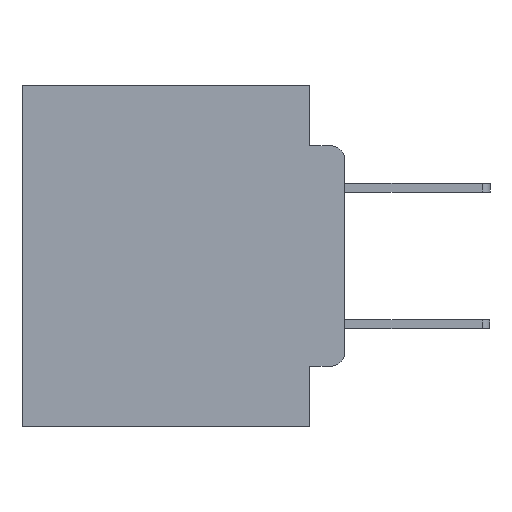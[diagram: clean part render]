
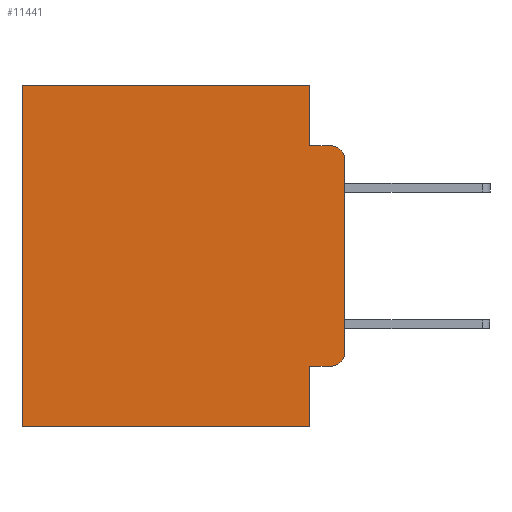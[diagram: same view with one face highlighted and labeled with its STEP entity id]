
A CAD part, left-side view. The second image highlights one B-rep face of the part: STEP entity #11441.
In plain terms, the highlighted planar face has unit normal (-1, 0, 0).
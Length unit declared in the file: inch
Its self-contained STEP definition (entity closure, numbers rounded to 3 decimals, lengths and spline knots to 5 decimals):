
#386 = VECTOR ( 'NONE', #3322, 39.37008 ) ;
#460 = AXIS2_PLACEMENT_3D ( 'NONE', #9773, #25426, #12042 ) ;
#721 = DIRECTION ( 'NONE',  ( 1., 0., 0. ) ) ;
#791 = ORIENTED_EDGE ( 'NONE', *, *, #3352, .T. ) ;
#1044 = DIRECTION ( 'NONE',  ( 0., 0., -1. ) ) ;
#1881 = DIRECTION ( 'NONE',  ( 0., -1., 0. ) ) ;
#1906 = DIRECTION ( 'NONE',  ( 0., 1., 0. ) ) ;
#2902 = ORIENTED_EDGE ( 'NONE', *, *, #4835, .T. ) ;
#3322 = DIRECTION ( 'NONE',  ( 0., -1., 0. ) ) ;
#3352 = EDGE_CURVE ( 'NONE', #27352, #16825, #17367, .T. ) ;
#3457 = VECTOR ( 'NONE', #28749, 39.37008 ) ;
#3898 = DIRECTION ( 'NONE',  ( 0., 0., -1. ) ) ;
#4165 = LINE ( 'NONE', #27867, #21397 ) ;
#4477 = VERTEX_POINT ( 'NONE', #10609 ) ;
#4835 = EDGE_CURVE ( 'NONE', #21523, #27352, #12340, .T. ) ;
#5110 = CARTESIAN_POINT ( 'NONE',  ( 0.298, 0., 0. ) ) ;
#5641 = ORIENTED_EDGE ( 'NONE', *, *, #12395, .F. ) ;
#6027 = ORIENTED_EDGE ( 'NONE', *, *, #15398, .T. ) ;
#6313 = VERTEX_POINT ( 'NONE', #15136 ) ;
#6376 = EDGE_CURVE ( 'NONE', #21523, #6313, #27283, .T. ) ;
#6821 = LINE ( 'NONE', #17628, #12786 ) ;
#7125 = CARTESIAN_POINT ( 'NONE',  ( 0.298, 0., -0.3915 ) ) ;
#7561 = CARTESIAN_POINT ( 'NONE',  ( 0.298, 0.051, 0. ) ) ;
#7868 = CARTESIAN_POINT ( 'NONE',  ( 0.298, 0.473, -0.5 ) ) ;
#8759 = AXIS2_PLACEMENT_3D ( 'NONE', #11425, #8792, #19826 ) ;
#8792 = DIRECTION ( 'NONE',  ( -1., 0., 0. ) ) ;
#9099 = DIRECTION ( 'NONE',  ( 0., 1., 0. ) ) ;
#9773 = CARTESIAN_POINT ( 'NONE',  ( 0.298, 0.02, -0.1085 ) ) ;
#10270 = CIRCLE ( 'NONE', #460, 0.02 ) ;
#10283 = ORIENTED_EDGE ( 'NONE', *, *, #10888, .T. ) ;
#10609 = CARTESIAN_POINT ( 'NONE',  ( 0.298, 0., -0.1085 ) ) ;
#10888 = EDGE_CURVE ( 'NONE', #22873, #23350, #4165, .T. ) ;
#11372 = ORIENTED_EDGE ( 'NONE', *, *, #20345, .F. ) ;
#11425 = CARTESIAN_POINT ( 'NONE',  ( 0.298, 0.02, -0.3915 ) ) ;
#11441 = ADVANCED_FACE ( 'NONE', ( #13282 ), #27559, .F. ) ;
#11449 = VECTOR ( 'NONE', #1906, 39.37008 ) ;
#11831 = VECTOR ( 'NONE', #3898, 39.37008 ) ;
#12042 = DIRECTION ( 'NONE',  ( 0., 0., -1. ) ) ;
#12340 = LINE ( 'NONE', #14518, #386 ) ;
#12395 = EDGE_CURVE ( 'NONE', #15756, #24917, #23702, .T. ) ;
#12786 = VECTOR ( 'NONE', #1881, 39.37008 ) ;
#13282 = FACE_OUTER_BOUND ( 'NONE', #25445, .T. ) ;
#13897 = EDGE_CURVE ( 'NONE', #24917, #16363, #6821, .T. ) ;
#14015 = ORIENTED_EDGE ( 'NONE', *, *, #20164, .T. ) ;
#14198 = CARTESIAN_POINT ( 'NONE',  ( 0.298, 0.02, -0.0885 ) ) ;
#14518 = CARTESIAN_POINT ( 'NONE',  ( 0.298, 0.051, -0.4115 ) ) ;
#14847 = ORIENTED_EDGE ( 'NONE', *, *, #6376, .F. ) ;
#15136 = CARTESIAN_POINT ( 'NONE',  ( 0.298, 0.051, -0.5 ) ) ;
#15398 = EDGE_CURVE ( 'NONE', #4477, #16363, #10270, .T. ) ;
#15756 = VERTEX_POINT ( 'NONE', #7561 ) ;
#15856 = CARTESIAN_POINT ( 'NONE',  ( 0.298, 0., -0.5 ) ) ;
#16363 = VERTEX_POINT ( 'NONE', #14198 ) ;
#16438 = DIRECTION ( 'NONE',  ( 0., 0., -1. ) ) ;
#16549 = CARTESIAN_POINT ( 'NONE',  ( 0.298, 0.051, -0.0885 ) ) ;
#16825 = VERTEX_POINT ( 'NONE', #7125 ) ;
#17367 = CIRCLE ( 'NONE', #8759, 0.02 ) ;
#17628 = CARTESIAN_POINT ( 'NONE',  ( 0.298, 0.051, -0.0885 ) ) ;
#18712 = ORIENTED_EDGE ( 'NONE', *, *, #22890, .F. ) ;
#18845 = LINE ( 'NONE', #22023, #11449 ) ;
#19181 = VECTOR ( 'NONE', #9099, 39.37008 ) ;
#19659 = CARTESIAN_POINT ( 'NONE',  ( 0.298, 0.051, 0. ) ) ;
#19826 = DIRECTION ( 'NONE',  ( 0., 0., -1. ) ) ;
#19893 = LINE ( 'NONE', #15856, #19181 ) ;
#20164 = EDGE_CURVE ( 'NONE', #15756, #22873, #18845, .T. ) ;
#20345 = EDGE_CURVE ( 'NONE', #6313, #23350, #19893, .T. ) ;
#20435 = VECTOR ( 'NONE', #28684, 39.37008 ) ;
#21119 = LINE ( 'NONE', #26500, #20435 ) ;
#21177 = ORIENTED_EDGE ( 'NONE', *, *, #13897, .F. ) ;
#21397 = VECTOR ( 'NONE', #1044, 39.37008 ) ;
#21523 = VERTEX_POINT ( 'NONE', #26732 ) ;
#22023 = CARTESIAN_POINT ( 'NONE',  ( 0.298, 0., 0. ) ) ;
#22873 = VERTEX_POINT ( 'NONE', #24133 ) ;
#22890 = EDGE_CURVE ( 'NONE', #4477, #16825, #21119, .T. ) ;
#23350 = VERTEX_POINT ( 'NONE', #7868 ) ;
#23702 = LINE ( 'NONE', #19659, #11831 ) ;
#24133 = CARTESIAN_POINT ( 'NONE',  ( 0.298, 0.473, 0. ) ) ;
#24917 = VERTEX_POINT ( 'NONE', #16549 ) ;
#25426 = DIRECTION ( 'NONE',  ( -1., 0., 0. ) ) ;
#25445 = EDGE_LOOP ( 'NONE', ( #18712, #6027, #21177, #5641, #14015, #10283, #11372, #14847, #2902, #791 ) ) ;
#26144 = AXIS2_PLACEMENT_3D ( 'NONE', #5110, #721, #16438 ) ;
#26500 = CARTESIAN_POINT ( 'NONE',  ( 0.298, 0., 0. ) ) ;
#26569 = CARTESIAN_POINT ( 'NONE',  ( 0.298, 0.051, 0. ) ) ;
#26732 = CARTESIAN_POINT ( 'NONE',  ( 0.298, 0.051, -0.4115 ) ) ;
#27283 = LINE ( 'NONE', #26569, #3457 ) ;
#27339 = CARTESIAN_POINT ( 'NONE',  ( 0.298, 0.02, -0.4115 ) ) ;
#27352 = VERTEX_POINT ( 'NONE', #27339 ) ;
#27559 = PLANE ( 'NONE',  #26144 ) ;
#27867 = CARTESIAN_POINT ( 'NONE',  ( 0.298, 0.473, 0. ) ) ;
#28684 = DIRECTION ( 'NONE',  ( 0., 0., -1. ) ) ;
#28749 = DIRECTION ( 'NONE',  ( 0., 0., -1. ) ) ;
